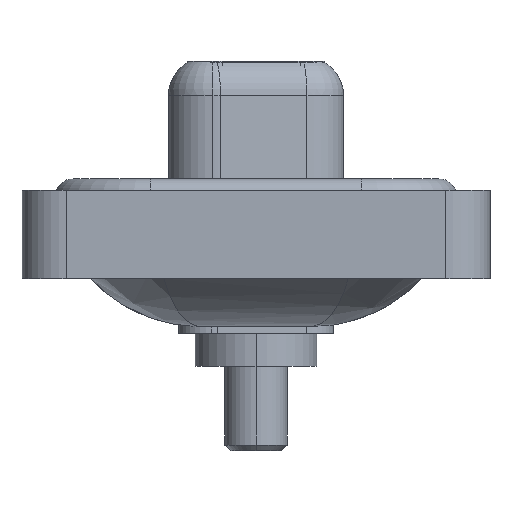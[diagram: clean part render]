
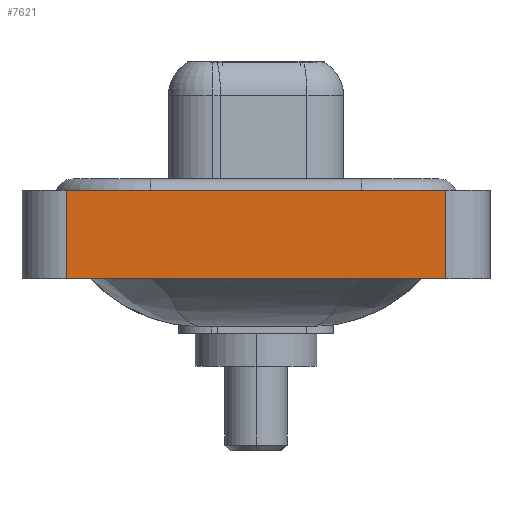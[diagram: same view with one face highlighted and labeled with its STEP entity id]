
A CAD part, left-side view. The second image highlights one B-rep face of the part: STEP entity #7621.
In plain terms, the highlighted planar face has unit normal (-1, 0, 0).
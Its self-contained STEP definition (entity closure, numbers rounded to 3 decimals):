
#1071 = ORIENTED_EDGE ( 'NONE', *, *, #3085, .T. ) ;
#1213 = EDGE_CURVE ( 'NONE', #9441, #10000, #13296, .T. ) ;
#1231 = EDGE_CURVE ( 'NONE', #10309, #13531, #7299, .T. ) ;
#1349 = CARTESIAN_POINT ( 'NONE',  ( -7.25, 8.55, 0.4 ) ) ;
#1683 = ORIENTED_EDGE ( 'NONE', *, *, #1213, .T. ) ;
#1736 = AXIS2_PLACEMENT_3D ( 'NONE', #15317, #4349, #11551 ) ;
#2428 = DIRECTION ( 'NONE',  ( 0., 0., 1. ) ) ;
#3085 = EDGE_CURVE ( 'NONE', #10000, #13531, #10875, .T. ) ;
#3885 = DIRECTION ( 'NONE',  ( 0., -1., 0. ) ) ;
#4349 = DIRECTION ( 'NONE',  ( -1., 0., 0. ) ) ;
#4490 = FACE_OUTER_BOUND ( 'NONE', #9572, .T. ) ;
#4613 = CARTESIAN_POINT ( 'NONE',  ( -7.25, -8.55, -3.6 ) ) ;
#4838 = CARTESIAN_POINT ( 'NONE',  ( -7.25, -8.55, 0.4 ) ) ;
#4848 = DIRECTION ( 'NONE',  ( 0., 0., 1. ) ) ;
#5841 = PLANE ( 'NONE',  #1736 ) ;
#6440 = EDGE_CURVE ( 'NONE', #9441, #10309, #10673, .T. ) ;
#7185 = CARTESIAN_POINT ( 'NONE',  ( -7.25, 8.55, -3.6 ) ) ;
#7299 = LINE ( 'NONE', #4838, #11578 ) ;
#7621 = ADVANCED_FACE ( 'NONE', ( #4490 ), #5841, .T. ) ;
#8083 = ORIENTED_EDGE ( 'NONE', *, *, #1231, .F. ) ;
#8235 = CARTESIAN_POINT ( 'NONE',  ( -7.25, -8.55, 0.4 ) ) ;
#8549 = VECTOR ( 'NONE', #10777, 1000. ) ;
#9284 = CARTESIAN_POINT ( 'NONE',  ( -7.25, -8.55, -3.6 ) ) ;
#9441 = VERTEX_POINT ( 'NONE', #10255 ) ;
#9572 = EDGE_LOOP ( 'NONE', ( #1071, #8083, #13372, #1683 ) ) ;
#10000 = VERTEX_POINT ( 'NONE', #9284 ) ;
#10081 = VECTOR ( 'NONE', #4848, 1000. ) ;
#10255 = CARTESIAN_POINT ( 'NONE',  ( -7.25, 8.55, -3.6 ) ) ;
#10309 = VERTEX_POINT ( 'NONE', #1349 ) ;
#10673 = LINE ( 'NONE', #7185, #14761 ) ;
#10777 = DIRECTION ( 'NONE',  ( 0., -1., 0. ) ) ;
#10875 = LINE ( 'NONE', #4613, #10081 ) ;
#11551 = DIRECTION ( 'NONE',  ( 0., 0., 1. ) ) ;
#11578 = VECTOR ( 'NONE', #3885, 1000. ) ;
#12288 = CARTESIAN_POINT ( 'NONE',  ( -7.25, -8.55, -3.6 ) ) ;
#13296 = LINE ( 'NONE', #12288, #8549 ) ;
#13372 = ORIENTED_EDGE ( 'NONE', *, *, #6440, .F. ) ;
#13531 = VERTEX_POINT ( 'NONE', #8235 ) ;
#14761 = VECTOR ( 'NONE', #2428, 1000. ) ;
#15317 = CARTESIAN_POINT ( 'NONE',  ( -7.25, -8.55, -3.6 ) ) ;
